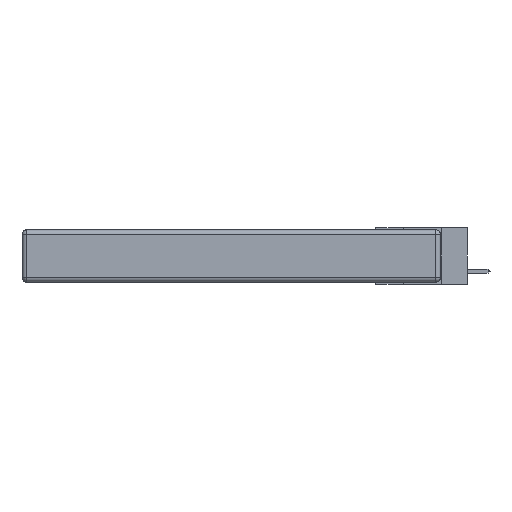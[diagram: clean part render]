
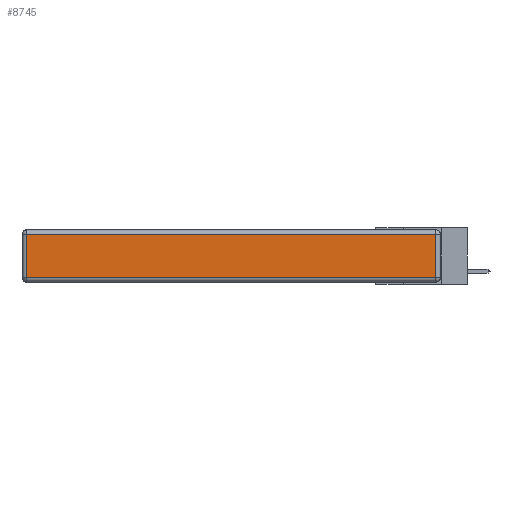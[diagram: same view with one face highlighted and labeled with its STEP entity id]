
A CAD part, left-side view. The second image highlights one B-rep face of the part: STEP entity #8745.
In plain terms, the highlighted planar face has unit normal (-1, 0, 0).
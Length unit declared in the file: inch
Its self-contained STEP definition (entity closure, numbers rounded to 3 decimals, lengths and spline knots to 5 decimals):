
#1837 = CARTESIAN_POINT ( 'NONE',  ( 0., 2.75, -0.03 ) ) ;
#2076 = DIRECTION ( 'NONE',  ( 0., -1., 0. ) ) ;
#2326 = VERTEX_POINT ( 'NONE', #9076 ) ;
#2464 = EDGE_CURVE ( 'NONE', #6677, #2326, #6814, .T. ) ;
#3627 = VECTOR ( 'NONE', #4337, 39.37008 ) ;
#3761 = LINE ( 'NONE', #4833, #11642 ) ;
#3796 = DIRECTION ( 'NONE',  ( 0., 1., 0. ) ) ;
#4085 = CARTESIAN_POINT ( 'NONE',  ( 0., 2.72, -0.03 ) ) ;
#4222 = CARTESIAN_POINT ( 'NONE',  ( 0., 2.72, -0.343 ) ) ;
#4337 = DIRECTION ( 'NONE',  ( 0., 0., -1. ) ) ;
#4447 = VERTEX_POINT ( 'NONE', #13194 ) ;
#4833 = CARTESIAN_POINT ( 'NONE',  ( 0., 0., -0.313 ) ) ;
#5597 = DIRECTION ( 'NONE',  ( -1., 0., 0. ) ) ;
#6677 = VERTEX_POINT ( 'NONE', #15368 ) ;
#6793 = LINE ( 'NONE', #1837, #12099 ) ;
#6814 = LINE ( 'NONE', #16115, #13157 ) ;
#8003 = AXIS2_PLACEMENT_3D ( 'NONE', #9588, #5597, #9342 ) ;
#8194 = EDGE_CURVE ( 'NONE', #16044, #4447, #14442, .T. ) ;
#8258 = PLANE ( 'NONE',  #8003 ) ;
#8745 = ADVANCED_FACE ( 'NONE', ( #16007 ), #8258, .T. ) ;
#8792 = ORIENTED_EDGE ( 'NONE', *, *, #16379, .T. ) ;
#9076 = CARTESIAN_POINT ( 'NONE',  ( 0., 0.03, -0.03 ) ) ;
#9325 = ORIENTED_EDGE ( 'NONE', *, *, #2464, .T. ) ;
#9342 = DIRECTION ( 'NONE',  ( 0., 0., 1. ) ) ;
#9525 = ORIENTED_EDGE ( 'NONE', *, *, #8194, .T. ) ;
#9588 = CARTESIAN_POINT ( 'NONE',  ( 0., 0., -0.343 ) ) ;
#10718 = ORIENTED_EDGE ( 'NONE', *, *, #15438, .T. ) ;
#10840 = DIRECTION ( 'NONE',  ( 0., 0., 1. ) ) ;
#11642 = VECTOR ( 'NONE', #2076, 39.37008 ) ;
#12099 = VECTOR ( 'NONE', #3796, 39.37008 ) ;
#13157 = VECTOR ( 'NONE', #10840, 39.37008 ) ;
#13194 = CARTESIAN_POINT ( 'NONE',  ( 0., 2.72, -0.313 ) ) ;
#13430 = EDGE_LOOP ( 'NONE', ( #8792, #9325, #10718, #9525 ) ) ;
#14442 = LINE ( 'NONE', #4222, #3627 ) ;
#15368 = CARTESIAN_POINT ( 'NONE',  ( 0., 0.03, -0.313 ) ) ;
#15438 = EDGE_CURVE ( 'NONE', #2326, #16044, #6793, .T. ) ;
#16007 = FACE_OUTER_BOUND ( 'NONE', #13430, .T. ) ;
#16044 = VERTEX_POINT ( 'NONE', #4085 ) ;
#16115 = CARTESIAN_POINT ( 'NONE',  ( 0., 0.03, -0.343 ) ) ;
#16379 = EDGE_CURVE ( 'NONE', #4447, #6677, #3761, .T. ) ;
